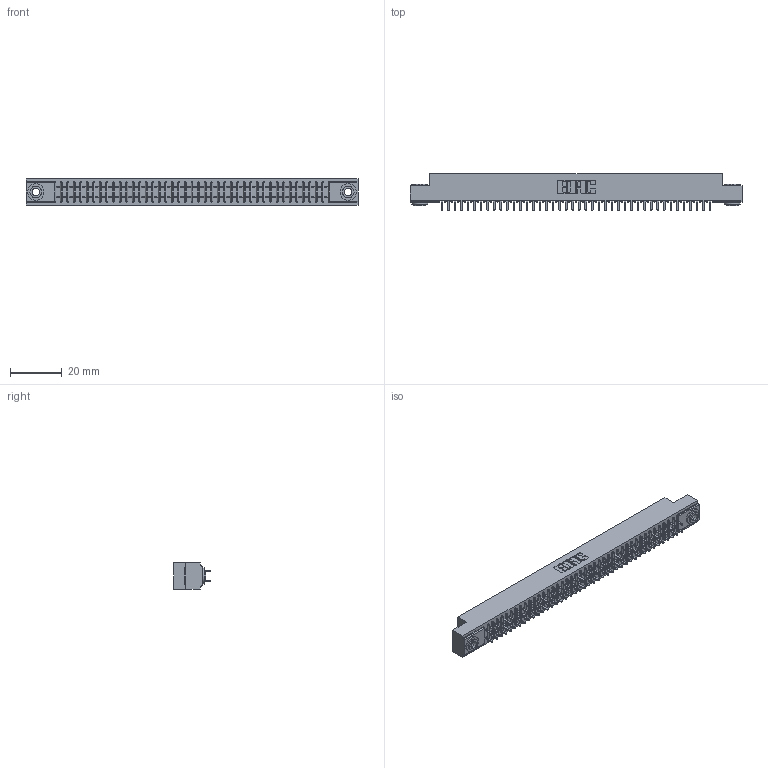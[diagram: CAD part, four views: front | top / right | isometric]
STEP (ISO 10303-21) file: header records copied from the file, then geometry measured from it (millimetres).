
FILE_DESCRIPTION (( 'STEP AP203' ), '1' );
FILE_NAME ('341-084-520-203.STEP', '2018-08-07T22:30:36', ( '' ), ( '' ), 'SwSTEP 2.0', 'SolidWorks 2016', '' );
FILE_SCHEMA (( 'CONFIG_CONTROL_DESIGN' ));
Length unit declared in the file: inch
Products named in the file (4): 341 Part_.156 (3.96) Dia Mounting Holes; 341-292-001_341-292-120; 345-250-002_345-250-002-102; 341-084-520-203
Assembly tree (87 placements, depth 2):
  341-084-520-203
    341 Part_.156 (3.96) Dia Mounting Holes
    341-292-001_341-292-120  x84
    345-250-002_345-250-002-102  x2
Bounding box: 128.91 x 14.27 x 10.16 mm (x, y, z)
Volume: 9523.6 mm3; surface area: 17070.9 mm2
Topology: 87 solids, 87 shells, 5712 faces, 16514 edges, 10694 vertices
Faces by surface type: plane 3452, cylinder 2084, sphere 86, torus 82, cone 8
Entity records: 51894 total; most frequent: CARTESIAN_POINT 8607, ORIENTED_EDGE 8544, DIRECTION 8368, EDGE_CURVE 4272, LINE 3442, VECTOR 3442, VERTEX_POINT 2702, AXIS2_PLACEMENT_3D 2463
